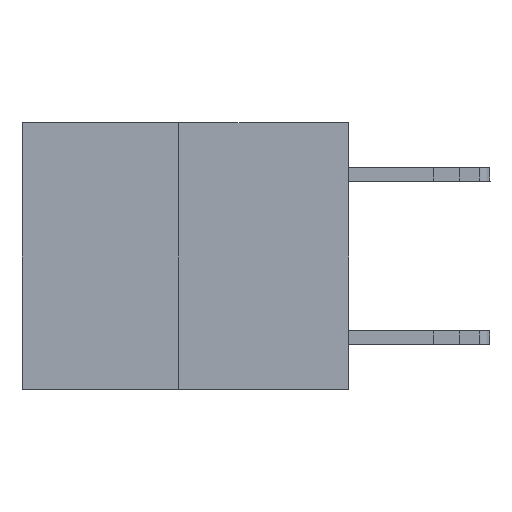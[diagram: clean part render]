
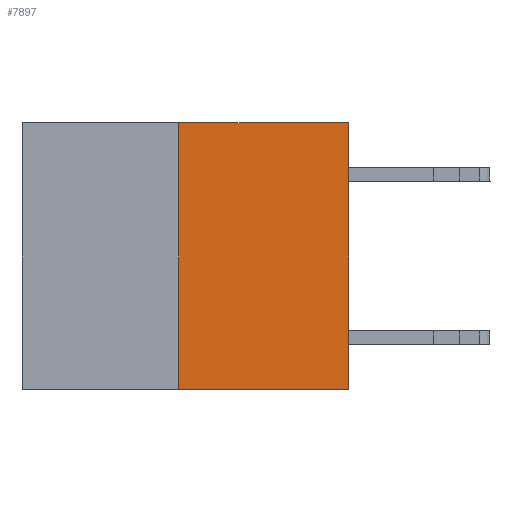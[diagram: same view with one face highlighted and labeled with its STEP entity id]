
A CAD part, left-side view. The second image highlights one B-rep face of the part: STEP entity #7897.
In plain terms, the highlighted planar face has unit normal (-1, 0, 0).
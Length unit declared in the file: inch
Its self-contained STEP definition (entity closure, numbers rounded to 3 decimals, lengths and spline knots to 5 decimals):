
#951 = CARTESIAN_POINT ( 'NONE',  ( 0., 0., 0. ) ) ;
#973 = VERTEX_POINT ( 'NONE', #2554 ) ;
#1611 = CARTESIAN_POINT ( 'NONE',  ( 0., 0.312, -0.49 ) ) ;
#1870 = DIRECTION ( 'NONE',  ( 0., -1., 0. ) ) ;
#1961 = EDGE_CURVE ( 'NONE', #973, #13817, #22069, .T. ) ;
#2328 = CARTESIAN_POINT ( 'NONE',  ( 0., 0.312, 0. ) ) ;
#2554 = CARTESIAN_POINT ( 'NONE',  ( 0., 0.312, -0.49 ) ) ;
#2643 = CARTESIAN_POINT ( 'NONE',  ( 0., 0., -0.49 ) ) ;
#2709 = ORIENTED_EDGE ( 'NONE', *, *, #12901, .F. ) ;
#3043 = EDGE_CURVE ( 'NONE', #973, #9933, #23458, .T. ) ;
#3423 = DIRECTION ( 'NONE',  ( 0., -1., 0. ) ) ;
#3580 = VECTOR ( 'NONE', #3423, 39.37008 ) ;
#3784 = FACE_OUTER_BOUND ( 'NONE', #11590, .T. ) ;
#4115 = ORIENTED_EDGE ( 'NONE', *, *, #11196, .T. ) ;
#4995 = CARTESIAN_POINT ( 'NONE',  ( 0., 0.6, 0. ) ) ;
#5361 = PLANE ( 'NONE',  #18629 ) ;
#5993 = CARTESIAN_POINT ( 'NONE',  ( 0., 0., 0. ) ) ;
#6360 = ORIENTED_EDGE ( 'NONE', *, *, #3043, .T. ) ;
#6931 = ORIENTED_EDGE ( 'NONE', *, *, #1961, .F. ) ;
#7487 = VECTOR ( 'NONE', #1870, 39.37008 ) ;
#7897 = ADVANCED_FACE ( 'NONE', ( #3784 ), #5361, .F. ) ;
#9295 = VECTOR ( 'NONE', #17286, 39.37008 ) ;
#9933 = VERTEX_POINT ( 'NONE', #2643 ) ;
#10555 = DIRECTION ( 'NONE',  ( 0., 0., 1. ) ) ;
#10753 = CARTESIAN_POINT ( 'NONE',  ( 0., 0.6, 0. ) ) ;
#10890 = CARTESIAN_POINT ( 'NONE',  ( 0., 0.6, -0.49 ) ) ;
#11016 = VERTEX_POINT ( 'NONE', #5993 ) ;
#11196 = EDGE_CURVE ( 'NONE', #9933, #11016, #19002, .T. ) ;
#11590 = EDGE_LOOP ( 'NONE', ( #6931, #6360, #4115, #2709 ) ) ;
#11818 = LINE ( 'NONE', #4995, #3580 ) ;
#12368 = VECTOR ( 'NONE', #10555, 39.37008 ) ;
#12574 = DIRECTION ( 'NONE',  ( 1., 0., 0. ) ) ;
#12901 = EDGE_CURVE ( 'NONE', #13817, #11016, #11818, .T. ) ;
#13817 = VERTEX_POINT ( 'NONE', #2328 ) ;
#17286 = DIRECTION ( 'NONE',  ( 0., 0., 1. ) ) ;
#18629 = AXIS2_PLACEMENT_3D ( 'NONE', #10753, #12574, #23443 ) ;
#19002 = LINE ( 'NONE', #951, #9295 ) ;
#22069 = LINE ( 'NONE', #1611, #12368 ) ;
#23443 = DIRECTION ( 'NONE',  ( 0., 0., -1. ) ) ;
#23458 = LINE ( 'NONE', #10890, #7487 ) ;
